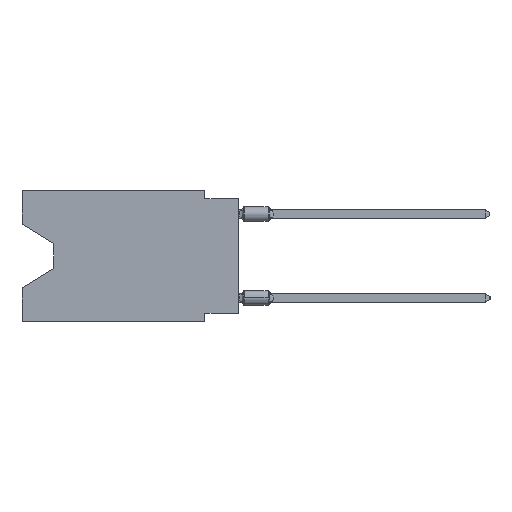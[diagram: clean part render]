
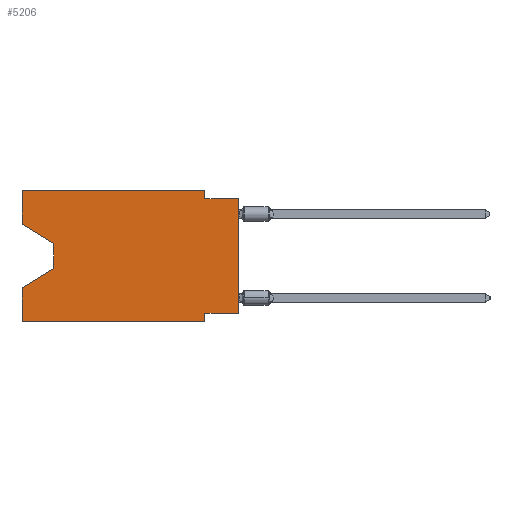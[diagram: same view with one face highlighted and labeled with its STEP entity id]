
A CAD part, left-side view. The second image highlights one B-rep face of the part: STEP entity #5206.
In plain terms, the highlighted planar face has unit normal (-1, 0, 0).
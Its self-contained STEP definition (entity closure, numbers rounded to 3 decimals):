
#833 = DIRECTION ( 'NONE',  ( 0., 0., 1. ) ) ;
#1161 = CARTESIAN_POINT ( 'NONE',  ( 0., 2.54, -9.906 ) ) ;
#1526 = CARTESIAN_POINT ( 'NONE',  ( 0., 13.97, -5.893 ) ) ;
#1639 = VERTEX_POINT ( 'NONE', #18037 ) ;
#1860 = DIRECTION ( 'NONE',  ( 0., -1., 0. ) ) ;
#2470 = CARTESIAN_POINT ( 'NONE',  ( 0., 16.383, 0. ) ) ;
#2872 = DIRECTION ( 'NONE',  ( 0., -0.855, -0.519 ) ) ;
#3275 = ORIENTED_EDGE ( 'NONE', *, *, #28901, .T. ) ;
#3368 = LINE ( 'NONE', #15532, #18133 ) ;
#4275 = VERTEX_POINT ( 'NONE', #10429 ) ;
#4393 = LINE ( 'NONE', #36654, #31603 ) ;
#5001 = DIRECTION ( 'NONE',  ( 1., 0., 0. ) ) ;
#5206 = ADVANCED_FACE ( 'NONE', ( #7512 ), #19874, .F. ) ;
#5559 = ORIENTED_EDGE ( 'NONE', *, *, #38219, .F. ) ;
#6408 = LINE ( 'NONE', #33250, #30208 ) ;
#6786 = EDGE_CURVE ( 'NONE', #1639, #35755, #4393, .T. ) ;
#6839 = ORIENTED_EDGE ( 'NONE', *, *, #37883, .F. ) ;
#7050 = LINE ( 'NONE', #15759, #14941 ) ;
#7512 = FACE_OUTER_BOUND ( 'NONE', #14531, .T. ) ;
#8405 = CARTESIAN_POINT ( 'NONE',  ( 0., 2.54, 0. ) ) ;
#8476 = ORIENTED_EDGE ( 'NONE', *, *, #33400, .T. ) ;
#8884 = CARTESIAN_POINT ( 'NONE',  ( 0., 16.383, -2.546 ) ) ;
#9085 = DIRECTION ( 'NONE',  ( 0., -1., 0. ) ) ;
#10294 = EDGE_CURVE ( 'NONE', #21671, #17710, #34177, .T. ) ;
#10429 = CARTESIAN_POINT ( 'NONE',  ( 0., 16.383, 0. ) ) ;
#10917 = VECTOR ( 'NONE', #20259, 1000. ) ;
#11097 = VERTEX_POINT ( 'NONE', #27666 ) ;
#11301 = LINE ( 'NONE', #8405, #34885 ) ;
#11334 = ORIENTED_EDGE ( 'NONE', *, *, #27909, .T. ) ;
#11402 = CARTESIAN_POINT ( 'NONE',  ( 0., 16.383, 0. ) ) ;
#11899 = DIRECTION ( 'NONE',  ( 0., 0.855, -0.519 ) ) ;
#12468 = VERTEX_POINT ( 'NONE', #25528 ) ;
#14089 = DIRECTION ( 'NONE',  ( 0., 0., -1. ) ) ;
#14346 = VECTOR ( 'NONE', #11899, 1000. ) ;
#14487 = LINE ( 'NONE', #8884, #29229 ) ;
#14531 = EDGE_LOOP ( 'NONE', ( #11334, #27436, #3275, #32322, #8476, #15042, #28284, #24952, #14803, #16169, #6839, #5559 ) ) ;
#14803 = ORIENTED_EDGE ( 'NONE', *, *, #6786, .F. ) ;
#14941 = VECTOR ( 'NONE', #19030, 1000. ) ;
#14990 = CARTESIAN_POINT ( 'NONE',  ( 0., 13.97, -5.893 ) ) ;
#15042 = ORIENTED_EDGE ( 'NONE', *, *, #18826, .F. ) ;
#15532 = CARTESIAN_POINT ( 'NONE',  ( 0., 0., 0. ) ) ;
#15759 = CARTESIAN_POINT ( 'NONE',  ( 0., 13.97, -4.013 ) ) ;
#16169 = ORIENTED_EDGE ( 'NONE', *, *, #25636, .F. ) ;
#17582 = LINE ( 'NONE', #11402, #38220 ) ;
#17710 = VERTEX_POINT ( 'NONE', #23286 ) ;
#17790 = EDGE_CURVE ( 'NONE', #21671, #35755, #3368, .T. ) ;
#18037 = CARTESIAN_POINT ( 'NONE',  ( 0., 2.54, -0.635 ) ) ;
#18133 = VECTOR ( 'NONE', #833, 1000. ) ;
#18357 = CARTESIAN_POINT ( 'NONE',  ( 0., 0., -9.271 ) ) ;
#18826 = EDGE_CURVE ( 'NONE', #17710, #11097, #27650, .T. ) ;
#19030 = DIRECTION ( 'NONE',  ( 0., 0., -1. ) ) ;
#19041 = VERTEX_POINT ( 'NONE', #21432 ) ;
#19495 = CARTESIAN_POINT ( 'NONE',  ( 0., 0., -9.271 ) ) ;
#19874 = PLANE ( 'NONE',  #31803 ) ;
#20259 = DIRECTION ( 'NONE',  ( 0., 1., 0. ) ) ;
#20663 = DIRECTION ( 'NONE',  ( 0., 0., 1. ) ) ;
#21276 = DIRECTION ( 'NONE',  ( 0., -1., 0. ) ) ;
#21432 = CARTESIAN_POINT ( 'NONE',  ( 0., 16.383, -9.906 ) ) ;
#21444 = VERTEX_POINT ( 'NONE', #31323 ) ;
#21455 = EDGE_CURVE ( 'NONE', #19041, #22631, #37091, .T. ) ;
#21671 = VERTEX_POINT ( 'NONE', #18357 ) ;
#21852 = DIRECTION ( 'NONE',  ( 0., 0., -1. ) ) ;
#22631 = VERTEX_POINT ( 'NONE', #24775 ) ;
#23286 = CARTESIAN_POINT ( 'NONE',  ( 0., 2.54, -9.271 ) ) ;
#23371 = LINE ( 'NONE', #38049, #37730 ) ;
#24775 = CARTESIAN_POINT ( 'NONE',  ( 0., 16.383, -7.36 ) ) ;
#24952 = ORIENTED_EDGE ( 'NONE', *, *, #17790, .T. ) ;
#25528 = CARTESIAN_POINT ( 'NONE',  ( 0., 2.54, 0. ) ) ;
#25636 = EDGE_CURVE ( 'NONE', #12468, #1639, #11301, .T. ) ;
#26257 = VECTOR ( 'NONE', #37669, 1000. ) ;
#27436 = ORIENTED_EDGE ( 'NONE', *, *, #35699, .T. ) ;
#27650 = LINE ( 'NONE', #1161, #35460 ) ;
#27666 = CARTESIAN_POINT ( 'NONE',  ( 0., 2.54, -9.906 ) ) ;
#27909 = EDGE_CURVE ( 'NONE', #21444, #34159, #14487, .T. ) ;
#28284 = ORIENTED_EDGE ( 'NONE', *, *, #10294, .F. ) ;
#28701 = CARTESIAN_POINT ( 'NONE',  ( 0., 0., -0.635 ) ) ;
#28901 = EDGE_CURVE ( 'NONE', #29429, #22631, #32386, .T. ) ;
#29229 = VECTOR ( 'NONE', #2872, 1000. ) ;
#29429 = VERTEX_POINT ( 'NONE', #1526 ) ;
#30208 = VECTOR ( 'NONE', #21276, 1000. ) ;
#31323 = CARTESIAN_POINT ( 'NONE',  ( 0., 16.383, -2.546 ) ) ;
#31603 = VECTOR ( 'NONE', #1860, 1000. ) ;
#31803 = AXIS2_PLACEMENT_3D ( 'NONE', #2470, #5001, #14089 ) ;
#31976 = DIRECTION ( 'NONE',  ( 0., 0., -1. ) ) ;
#32322 = ORIENTED_EDGE ( 'NONE', *, *, #21455, .F. ) ;
#32386 = LINE ( 'NONE', #14990, #14346 ) ;
#33250 = CARTESIAN_POINT ( 'NONE',  ( 0., 16.383, 0. ) ) ;
#33400 = EDGE_CURVE ( 'NONE', #19041, #11097, #23371, .T. ) ;
#33564 = CARTESIAN_POINT ( 'NONE',  ( 0., 13.97, -4.013 ) ) ;
#34159 = VERTEX_POINT ( 'NONE', #33564 ) ;
#34177 = LINE ( 'NONE', #19495, #10917 ) ;
#34885 = VECTOR ( 'NONE', #31976, 1000. ) ;
#35460 = VECTOR ( 'NONE', #21852, 1000. ) ;
#35699 = EDGE_CURVE ( 'NONE', #34159, #29429, #7050, .T. ) ;
#35755 = VERTEX_POINT ( 'NONE', #28701 ) ;
#36654 = CARTESIAN_POINT ( 'NONE',  ( 0., 0., -0.635 ) ) ;
#37091 = LINE ( 'NONE', #37295, #26257 ) ;
#37295 = CARTESIAN_POINT ( 'NONE',  ( 0., 16.383, 0. ) ) ;
#37669 = DIRECTION ( 'NONE',  ( 0., 0., 1. ) ) ;
#37730 = VECTOR ( 'NONE', #9085, 1000. ) ;
#37883 = EDGE_CURVE ( 'NONE', #4275, #12468, #6408, .T. ) ;
#38049 = CARTESIAN_POINT ( 'NONE',  ( 0., 16.383, -9.906 ) ) ;
#38219 = EDGE_CURVE ( 'NONE', #21444, #4275, #17582, .T. ) ;
#38220 = VECTOR ( 'NONE', #20663, 1000. ) ;
